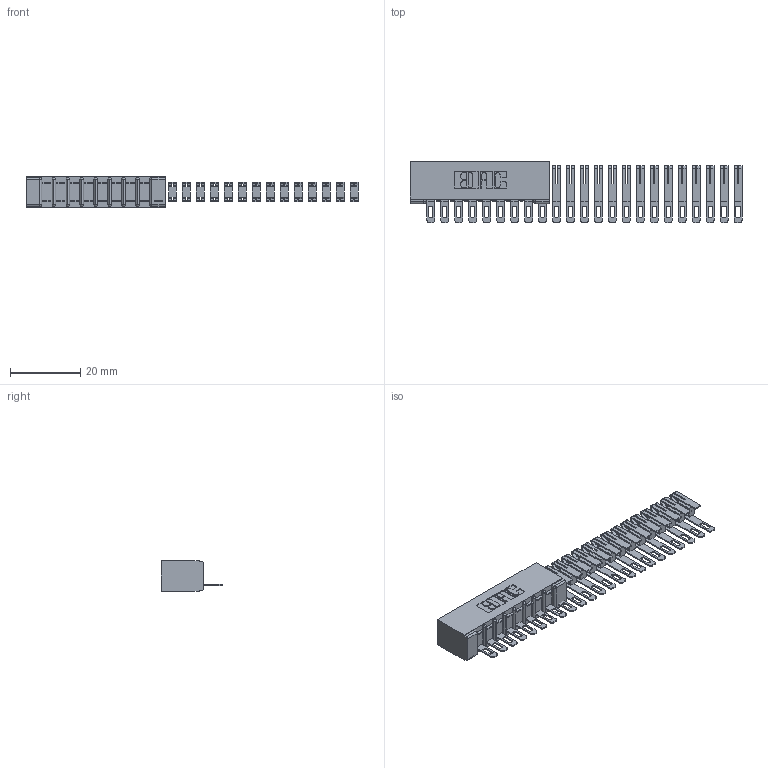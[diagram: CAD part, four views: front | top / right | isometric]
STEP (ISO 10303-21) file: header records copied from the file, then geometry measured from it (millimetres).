
FILE_DESCRIPTION (( 'STEP AP203' ), '1' );
FILE_NAME ('357-023-501-101.STEP', '2018-08-08T23:36:03', ( '' ), ( '' ), 'SwSTEP 2.0', 'SolidWorks 2016', '' );
FILE_SCHEMA (( 'CONFIG_CONTROL_DESIGN' ));
Length unit declared in the file: inch
Products named in the file (3): 307-290-002_501; 357-023-501-101; 307 Part_No Mounting Lugs
Assembly tree (24 placements, depth 2):
  357-023-501-101
    307 Part_No Mounting Lugs
    307-290-002_501  x23
Bounding box: 94.22 x 17.42 x 8.71 mm (x, y, z)
Volume: 3301.6 mm3; surface area: 8418.2 mm2
Topology: 24 solids, 24 shells, 1567 faces, 4813 edges, 3182 vertices
Faces by surface type: plane 898, cylinder 651, sphere 18
Entity records: 12046 total; most frequent: CARTESIAN_POINT 1959, DIRECTION 1937, ORIENTED_EDGE 1934, EDGE_CURVE 967, LINE 721, VECTOR 721, VERTEX_POINT 630, AXIS2_PLACEMENT_3D 608
